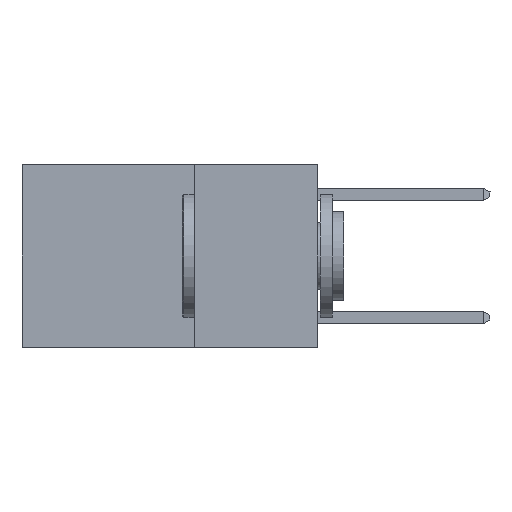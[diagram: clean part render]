
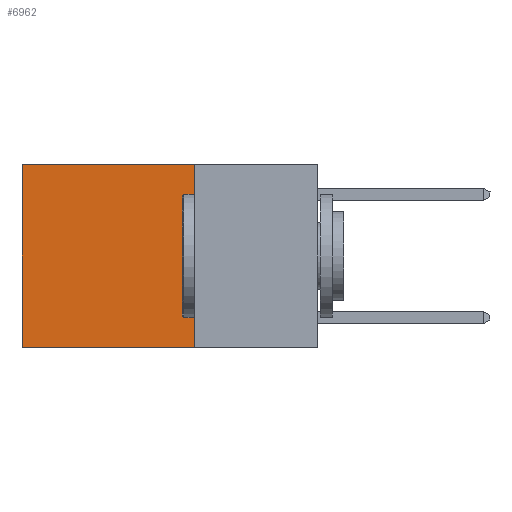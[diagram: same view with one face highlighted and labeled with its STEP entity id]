
A CAD part, left-side view. The second image highlights one B-rep face of the part: STEP entity #6962.
In plain terms, the highlighted planar face has unit normal (-1, 0, 0).
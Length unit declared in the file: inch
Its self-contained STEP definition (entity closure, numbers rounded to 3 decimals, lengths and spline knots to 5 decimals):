
#1249 = FACE_OUTER_BOUND ( 'NONE', #9983, .T. ) ;
#1293 = DIRECTION ( 'NONE',  ( 0., 1., 0. ) ) ;
#1444 = CARTESIAN_POINT ( 'NONE',  ( 0.2625, 0.6, 0. ) ) ;
#1483 = VERTEX_POINT ( 'NONE', #1444 ) ;
#1918 = PLANE ( 'NONE',  #11577 ) ;
#3792 = LINE ( 'NONE', #8267, #6528 ) ;
#3846 = CARTESIAN_POINT ( 'NONE',  ( 0.2625, 0.25, 0. ) ) ;
#4213 = VECTOR ( 'NONE', #12171, 39.37008 ) ;
#4300 = DIRECTION ( 'NONE',  ( 0., 0., -1. ) ) ;
#4610 = CARTESIAN_POINT ( 'NONE',  ( 0.2625, 0.6, 0. ) ) ;
#5195 = EDGE_CURVE ( 'NONE', #5758, #1483, #10907, .T. ) ;
#5271 = EDGE_CURVE ( 'NONE', #5758, #11460, #6215, .T. ) ;
#5369 = CARTESIAN_POINT ( 'NONE',  ( 0.2625, 0.25, 0. ) ) ;
#5697 = EDGE_CURVE ( 'NONE', #1483, #9870, #13218, .T. ) ;
#5758 = VERTEX_POINT ( 'NONE', #14056 ) ;
#5870 = DIRECTION ( 'NONE',  ( 0., 0., -1. ) ) ;
#6215 = LINE ( 'NONE', #5369, #12530 ) ;
#6528 = VECTOR ( 'NONE', #1293, 39.37008 ) ;
#6962 = ADVANCED_FACE ( 'NONE', ( #1249 ), #1918, .F. ) ;
#7271 = EDGE_CURVE ( 'NONE', #11460, #9870, #3792, .T. ) ;
#7351 = ORIENTED_EDGE ( 'NONE', *, *, #7271, .F. ) ;
#8267 = CARTESIAN_POINT ( 'NONE',  ( 0.2625, 0.25, -0.37 ) ) ;
#9870 = VERTEX_POINT ( 'NONE', #10368 ) ;
#9983 = EDGE_LOOP ( 'NONE', ( #14490, #7351, #11147, #10571 ) ) ;
#10236 = CARTESIAN_POINT ( 'NONE',  ( 0.2625, 0.25, 0. ) ) ;
#10368 = CARTESIAN_POINT ( 'NONE',  ( 0.2625, 0.6, -0.37 ) ) ;
#10571 = ORIENTED_EDGE ( 'NONE', *, *, #5195, .T. ) ;
#10907 = LINE ( 'NONE', #3846, #4213 ) ;
#11038 = CARTESIAN_POINT ( 'NONE',  ( 0.2625, 0.25, -0.37 ) ) ;
#11147 = ORIENTED_EDGE ( 'NONE', *, *, #5271, .F. ) ;
#11406 = DIRECTION ( 'NONE',  ( 1., 0., 0. ) ) ;
#11460 = VERTEX_POINT ( 'NONE', #11038 ) ;
#11577 = AXIS2_PLACEMENT_3D ( 'NONE', #10236, #11406, #4300 ) ;
#12171 = DIRECTION ( 'NONE',  ( 0., 1., 0. ) ) ;
#12530 = VECTOR ( 'NONE', #14763, 39.37008 ) ;
#12864 = VECTOR ( 'NONE', #5870, 39.37008 ) ;
#13218 = LINE ( 'NONE', #4610, #12864 ) ;
#14056 = CARTESIAN_POINT ( 'NONE',  ( 0.2625, 0.25, 0. ) ) ;
#14490 = ORIENTED_EDGE ( 'NONE', *, *, #5697, .T. ) ;
#14763 = DIRECTION ( 'NONE',  ( 0., 0., -1. ) ) ;
